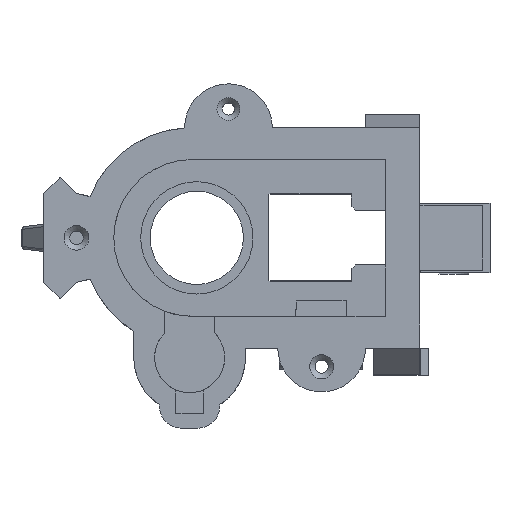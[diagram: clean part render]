
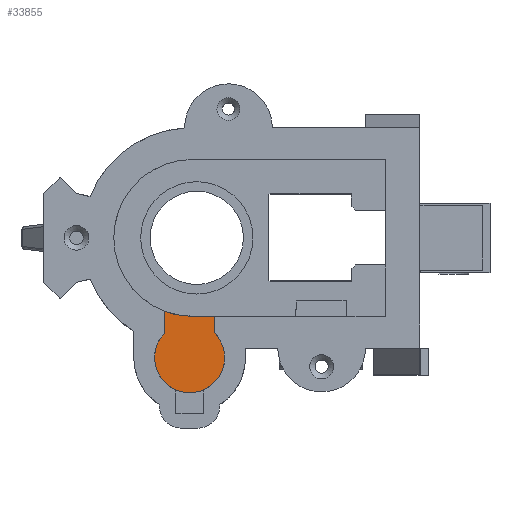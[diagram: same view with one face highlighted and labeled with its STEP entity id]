
A CAD part, left-side view. The second image highlights one B-rep face of the part: STEP entity #33855.
In plain terms, the highlighted planar face has unit normal (-1, 0, 0).
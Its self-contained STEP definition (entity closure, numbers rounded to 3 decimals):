
#7229 = PLANE('',#7230);
#7230 = AXIS2_PLACEMENT_3D('',#7231,#7232,#7233);
#7231 = CARTESIAN_POINT('',(-178.497,12.84,
    -14.3));
#7232 = DIRECTION('',(0.,0.,1.));
#7233 = DIRECTION('',(1.,0.,0.));
#7257 = PLANE('',#7258);
#7258 = AXIS2_PLACEMENT_3D('',#7259,#7260,#7261);
#7259 = CARTESIAN_POINT('',(-178.497,44.008,
    -17.302));
#7260 = DIRECTION('',(0.,-1.,0.));
#7261 = DIRECTION('',(0.,0.,-1.));
#7290 = CYLINDRICAL_SURFACE('',#7291,6.4);
#7291 = AXIS2_PLACEMENT_3D('',#7292,#7293,#7294);
#7292 = CARTESIAN_POINT('',(-178.497,48.508,-21.853));
#7293 = DIRECTION('',(-1.,0.,0.));
#7294 = DIRECTION('',(0.,0.,1.));
#7474 = PLANE('',#7475);
#7475 = AXIS2_PLACEMENT_3D('',#7476,#7477,#7478);
#7476 = CARTESIAN_POINT('',(-178.497,53.008,
    -17.302));
#7477 = DIRECTION('',(0.,-1.,0.));
#7478 = DIRECTION('',(0.,0.,-1.));
#7503 = CYLINDRICAL_SURFACE('',#7504,14.3);
#7504 = AXIS2_PLACEMENT_3D('',#7505,#7506,#7507);
#7505 = CARTESIAN_POINT('',(-178.497,48.04,0.));
#7506 = DIRECTION('',(-1.,0.,0.));
#7507 = DIRECTION('',(0.,0.,1.));
#20545 = EDGE_CURVE('',#20546,#20548,#20550,.T.);
#20546 = VERTEX_POINT('',#20547);
#20547 = CARTESIAN_POINT('',(-24.497,48.04,
    -14.3));
#20548 = VERTEX_POINT('',#20549);
#20549 = CARTESIAN_POINT('',(-24.497,44.008,
    -14.3));
#20550 = SURFACE_CURVE('',#20551,(#20555,#20562),.PCURVE_S1.);
#20551 = LINE('',#20552,#20553);
#20552 = CARTESIAN_POINT('',(-24.497,53.008,
    -14.3));
#20553 = VECTOR('',#20554,1.);
#20554 = DIRECTION('',(0.,-1.,0.));
#20555 = PCURVE('',#7229,#20556);
#20556 = DEFINITIONAL_REPRESENTATION('',(#20557),#20561);
#20557 = LINE('',#20558,#20559);
#20558 = CARTESIAN_POINT('',(154.,40.168));
#20559 = VECTOR('',#20560,1.);
#20560 = DIRECTION('',(0.,-1.));
#20561 = ( GEOMETRIC_REPRESENTATION_CONTEXT(2) 
PARAMETRIC_REPRESENTATION_CONTEXT() REPRESENTATION_CONTEXT('2D SPACE',''
  ) );
#20562 = PCURVE('',#20563,#20568);
#20563 = PLANE('',#20564);
#20564 = AXIS2_PLACEMENT_3D('',#20565,#20566,#20567);
#20565 = CARTESIAN_POINT('',(-24.497,53.008,
    -17.302));
#20566 = DIRECTION('',(1.,0.,0.));
#20567 = DIRECTION('',(0.,0.,-1.));
#20568 = DEFINITIONAL_REPRESENTATION('',(#20569),#20573);
#20569 = LINE('',#20570,#20571);
#20570 = CARTESIAN_POINT('',(-3.002,0.));
#20571 = VECTOR('',#20572,1.);
#20572 = DIRECTION('',(0.,-1.));
#20573 = ( GEOMETRIC_REPRESENTATION_CONTEXT(2) 
PARAMETRIC_REPRESENTATION_CONTEXT() REPRESENTATION_CONTEXT('2D SPACE',''
  ) );
#20990 = EDGE_CURVE('',#20548,#20991,#20993,.T.);
#20991 = VERTEX_POINT('',#20992);
#20992 = CARTESIAN_POINT('',(-24.497,44.008,
    -17.302));
#20993 = SURFACE_CURVE('',#20994,(#20998,#21005),.PCURVE_S1.);
#20994 = LINE('',#20995,#20996);
#20995 = CARTESIAN_POINT('',(-24.497,44.008,
    -17.302));
#20996 = VECTOR('',#20997,1.);
#20997 = DIRECTION('',(0.,0.,-1.));
#20998 = PCURVE('',#7257,#20999);
#20999 = DEFINITIONAL_REPRESENTATION('',(#21000),#21004);
#21000 = LINE('',#21001,#21002);
#21001 = CARTESIAN_POINT('',(0.,154.));
#21002 = VECTOR('',#21003,1.);
#21003 = DIRECTION('',(1.,0.));
#21004 = ( GEOMETRIC_REPRESENTATION_CONTEXT(2) 
PARAMETRIC_REPRESENTATION_CONTEXT() REPRESENTATION_CONTEXT('2D SPACE',''
  ) );
#21005 = PCURVE('',#20563,#21006);
#21006 = DEFINITIONAL_REPRESENTATION('',(#21007),#21011);
#21007 = LINE('',#21008,#21009);
#21008 = CARTESIAN_POINT('',(0.,-9.));
#21009 = VECTOR('',#21010,1.);
#21010 = DIRECTION('',(1.,0.));
#21011 = ( GEOMETRIC_REPRESENTATION_CONTEXT(2) 
PARAMETRIC_REPRESENTATION_CONTEXT() REPRESENTATION_CONTEXT('2D SPACE',''
  ) );
#21062 = VERTEX_POINT('',#21063);
#21063 = CARTESIAN_POINT('',(-24.497,53.008,
    -17.302));
#21106 = EDGE_CURVE('',#20991,#21062,#21107,.T.);
#21107 = SURFACE_CURVE('',#21108,(#21113,#21142),.PCURVE_S1.);
#21108 = CIRCLE('',#21109,6.4);
#21109 = AXIS2_PLACEMENT_3D('',#21110,#21111,#21112);
#21110 = CARTESIAN_POINT('',(-24.497,48.508,-21.853));
#21111 = DIRECTION('',(1.,0.,0.));
#21112 = DIRECTION('',(0.,0.,1.));
#21113 = PCURVE('',#7290,#21114);
#21114 = DEFINITIONAL_REPRESENTATION('',(#21115),#21141);
#21115 = B_SPLINE_CURVE_WITH_KNOTS('',3,(#21116,#21117,#21118,#21119,
    #21120,#21121,#21122,#21123,#21124,#21125,#21126,#21127,#21128,
    #21129,#21130,#21131,#21132,#21133,#21134,#21135,#21136,#21137,
    #21138,#21139,#21140),.UNSPECIFIED.,.F.,.F.,(4,1,1,1,1,1,1,1,1,1,1,1
    ,1,1,1,1,1,1,1,1,1,1,4),(0.78,0.994,1.209
    ,1.424,1.639,1.853,2.068,
    2.283,2.497,2.712,2.927,
    3.142,3.356,3.571,3.786,
    4.,4.215,4.43,4.645,
    4.859,5.074,5.289,5.503),
  .UNSPECIFIED.);
#21116 = CARTESIAN_POINT('',(5.503,-154.));
#21117 = CARTESIAN_POINT('',(5.432,-154.));
#21118 = CARTESIAN_POINT('',(5.289,-154.));
#21119 = CARTESIAN_POINT('',(5.074,-154.));
#21120 = CARTESIAN_POINT('',(4.859,-154.));
#21121 = CARTESIAN_POINT('',(4.645,-154.));
#21122 = CARTESIAN_POINT('',(4.43,-154.));
#21123 = CARTESIAN_POINT('',(4.215,-154.));
#21124 = CARTESIAN_POINT('',(4.,-154.));
#21125 = CARTESIAN_POINT('',(3.786,-154.));
#21126 = CARTESIAN_POINT('',(3.571,-154.));
#21127 = CARTESIAN_POINT('',(3.356,-154.));
#21128 = CARTESIAN_POINT('',(3.142,-154.));
#21129 = CARTESIAN_POINT('',(2.927,-154.));
#21130 = CARTESIAN_POINT('',(2.712,-154.));
#21131 = CARTESIAN_POINT('',(2.497,-154.));
#21132 = CARTESIAN_POINT('',(2.283,-154.));
#21133 = CARTESIAN_POINT('',(2.068,-154.));
#21134 = CARTESIAN_POINT('',(1.853,-154.));
#21135 = CARTESIAN_POINT('',(1.639,-154.));
#21136 = CARTESIAN_POINT('',(1.424,-154.));
#21137 = CARTESIAN_POINT('',(1.209,-154.));
#21138 = CARTESIAN_POINT('',(0.994,-154.));
#21139 = CARTESIAN_POINT('',(0.851,-154.));
#21140 = CARTESIAN_POINT('',(0.78,-154.));
#21141 = ( GEOMETRIC_REPRESENTATION_CONTEXT(2) 
PARAMETRIC_REPRESENTATION_CONTEXT() REPRESENTATION_CONTEXT('2D SPACE',''
  ) );
#21142 = PCURVE('',#20563,#21143);
#21143 = DEFINITIONAL_REPRESENTATION('',(#21144),#21148);
#21144 = CIRCLE('',#21145,6.4);
#21145 = AXIS2_PLACEMENT_2D('',#21146,#21147);
#21146 = CARTESIAN_POINT('',(4.551,-4.5));
#21147 = DIRECTION('',(-1.,0.));
#21148 = ( GEOMETRIC_REPRESENTATION_CONTEXT(2) 
PARAMETRIC_REPRESENTATION_CONTEXT() REPRESENTATION_CONTEXT('2D SPACE',''
  ) );
#21423 = EDGE_CURVE('',#21062,#21424,#21426,.T.);
#21424 = VERTEX_POINT('',#21425);
#21425 = CARTESIAN_POINT('',(-24.497,53.008,
    -13.409));
#21426 = SURFACE_CURVE('',#21427,(#21431,#21438),.PCURVE_S1.);
#21427 = LINE('',#21428,#21429);
#21428 = CARTESIAN_POINT('',(-24.497,53.008,
    -17.302));
#21429 = VECTOR('',#21430,1.);
#21430 = DIRECTION('',(0.,0.,1.));
#21431 = PCURVE('',#7474,#21432);
#21432 = DEFINITIONAL_REPRESENTATION('',(#21433),#21437);
#21433 = LINE('',#21434,#21435);
#21434 = CARTESIAN_POINT('',(0.,154.));
#21435 = VECTOR('',#21436,1.);
#21436 = DIRECTION('',(-1.,0.));
#21437 = ( GEOMETRIC_REPRESENTATION_CONTEXT(2) 
PARAMETRIC_REPRESENTATION_CONTEXT() REPRESENTATION_CONTEXT('2D SPACE',''
  ) );
#21438 = PCURVE('',#20563,#21439);
#21439 = DEFINITIONAL_REPRESENTATION('',(#21440),#21444);
#21440 = LINE('',#21441,#21442);
#21441 = CARTESIAN_POINT('',(0.,0.));
#21442 = VECTOR('',#21443,1.);
#21443 = DIRECTION('',(-1.,0.));
#21444 = ( GEOMETRIC_REPRESENTATION_CONTEXT(2) 
PARAMETRIC_REPRESENTATION_CONTEXT() REPRESENTATION_CONTEXT('2D SPACE',''
  ) );
#21589 = EDGE_CURVE('',#20546,#21424,#21590,.T.);
#21590 = SURFACE_CURVE('',#21591,(#21596,#21625),.PCURVE_S1.);
#21591 = CIRCLE('',#21592,14.3);
#21592 = AXIS2_PLACEMENT_3D('',#21593,#21594,#21595);
#21593 = CARTESIAN_POINT('',(-24.497,48.04,0.));
#21594 = DIRECTION('',(1.,0.,0.));
#21595 = DIRECTION('',(0.,0.,1.));
#21596 = PCURVE('',#7503,#21597);
#21597 = DEFINITIONAL_REPRESENTATION('',(#21598),#21624);
#21598 = B_SPLINE_CURVE_WITH_KNOTS('',3,(#21599,#21600,#21601,#21602,
    #21603,#21604,#21605,#21606,#21607,#21608,#21609,#21610,#21611,
    #21612,#21613,#21614,#21615,#21616,#21617,#21618,#21619,#21620,
    #21621,#21622,#21623),.UNSPECIFIED.,.F.,.F.,(4,1,1,1,1,1,1,1,1,1,1,1
    ,1,1,1,1,1,1,1,1,1,1,4),(3.142,3.158,3.174,
    3.19,3.206,3.222,3.238,
    3.254,3.271,3.287,3.303,
    3.319,3.335,3.351,3.367,
    3.384,3.4,3.416,3.432,
    3.448,3.464,3.48,3.496),
  .UNSPECIFIED.);
#21599 = CARTESIAN_POINT('',(3.142,-154.));
#21600 = CARTESIAN_POINT('',(3.136,-154.));
#21601 = CARTESIAN_POINT('',(3.125,-154.));
#21602 = CARTESIAN_POINT('',(3.109,-154.));
#21603 = CARTESIAN_POINT('',(3.093,-154.));
#21604 = CARTESIAN_POINT('',(3.077,-154.));
#21605 = CARTESIAN_POINT('',(3.061,-154.));
#21606 = CARTESIAN_POINT('',(3.045,-154.));
#21607 = CARTESIAN_POINT('',(3.029,-154.));
#21608 = CARTESIAN_POINT('',(3.013,-154.));
#21609 = CARTESIAN_POINT('',(2.996,-154.));
#21610 = CARTESIAN_POINT('',(2.98,-154.));
#21611 = CARTESIAN_POINT('',(2.964,-154.));
#21612 = CARTESIAN_POINT('',(2.948,-154.));
#21613 = CARTESIAN_POINT('',(2.932,-154.));
#21614 = CARTESIAN_POINT('',(2.916,-154.));
#21615 = CARTESIAN_POINT('',(2.9,-154.));
#21616 = CARTESIAN_POINT('',(2.884,-154.));
#21617 = CARTESIAN_POINT('',(2.867,-154.));
#21618 = CARTESIAN_POINT('',(2.851,-154.));
#21619 = CARTESIAN_POINT('',(2.835,-154.));
#21620 = CARTESIAN_POINT('',(2.819,-154.));
#21621 = CARTESIAN_POINT('',(2.803,-154.));
#21622 = CARTESIAN_POINT('',(2.792,-154.));
#21623 = CARTESIAN_POINT('',(2.787,-154.));
#21624 = ( GEOMETRIC_REPRESENTATION_CONTEXT(2) 
PARAMETRIC_REPRESENTATION_CONTEXT() REPRESENTATION_CONTEXT('2D SPACE',''
  ) );
#21625 = PCURVE('',#20563,#21626);
#21626 = DEFINITIONAL_REPRESENTATION('',(#21627),#21631);
#21627 = CIRCLE('',#21628,14.3);
#21628 = AXIS2_PLACEMENT_2D('',#21629,#21630);
#21629 = CARTESIAN_POINT('',(-17.302,-4.968));
#21630 = DIRECTION('',(-1.,0.));
#21631 = ( GEOMETRIC_REPRESENTATION_CONTEXT(2) 
PARAMETRIC_REPRESENTATION_CONTEXT() REPRESENTATION_CONTEXT('2D SPACE',''
  ) );
#33855 = ADVANCED_FACE('',(#33856),#20563,.F.);
#33856 = FACE_BOUND('',#33857,.T.);
#33857 = EDGE_LOOP('',(#33858,#33859,#33860,#33861,#33862));
#33858 = ORIENTED_EDGE('',*,*,#20990,.F.);
#33859 = ORIENTED_EDGE('',*,*,#20545,.F.);
#33860 = ORIENTED_EDGE('',*,*,#21589,.T.);
#33861 = ORIENTED_EDGE('',*,*,#21423,.F.);
#33862 = ORIENTED_EDGE('',*,*,#21106,.F.);
